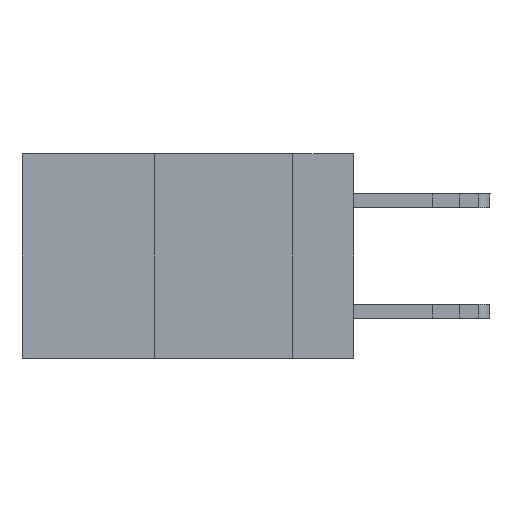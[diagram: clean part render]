
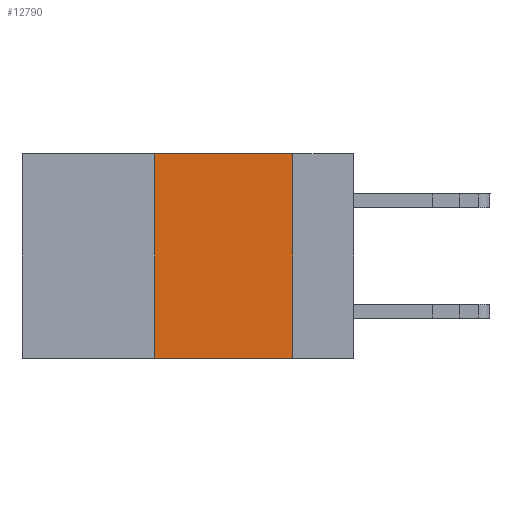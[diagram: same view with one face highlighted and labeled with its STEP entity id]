
A CAD part, left-side view. The second image highlights one B-rep face of the part: STEP entity #12790.
In plain terms, the highlighted planar face has unit normal (-1, 0, 0).
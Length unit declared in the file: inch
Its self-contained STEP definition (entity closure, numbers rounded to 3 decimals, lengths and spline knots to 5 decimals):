
#268 = CARTESIAN_POINT ( 'NONE',  ( 0., 0.36, 0. ) ) ;
#321 = FACE_OUTER_BOUND ( 'NONE', #9798, .T. ) ;
#323 = DIRECTION ( 'NONE',  ( 0., 0., 1. ) ) ;
#873 = ORIENTED_EDGE ( 'NONE', *, *, #4966, .F. ) ;
#1254 = EDGE_CURVE ( 'NONE', #4340, #8443, #14075, .T. ) ;
#1696 = EDGE_CURVE ( 'NONE', #13185, #4340, #14829, .T. ) ;
#3400 = LINE ( 'NONE', #268, #8341 ) ;
#4340 = VERTEX_POINT ( 'NONE', #11667 ) ;
#4399 = EDGE_CURVE ( 'NONE', #11257, #8443, #13982, .T. ) ;
#4766 = CARTESIAN_POINT ( 'NONE',  ( 0., 0.36, 0. ) ) ;
#4966 = EDGE_CURVE ( 'NONE', #11257, #13185, #3400, .T. ) ;
#5517 = DIRECTION ( 'NONE',  ( 0., 0., -1. ) ) ;
#5596 = DIRECTION ( 'NONE',  ( 1., 0., 0. ) ) ;
#7841 = VECTOR ( 'NONE', #8449, 39.37008 ) ;
#8010 = CARTESIAN_POINT ( 'NONE',  ( 0., 0.6, -0.37 ) ) ;
#8341 = VECTOR ( 'NONE', #323, 39.37008 ) ;
#8443 = VERTEX_POINT ( 'NONE', #10993 ) ;
#8449 = DIRECTION ( 'NONE',  ( 0., -1., 0. ) ) ;
#8572 = ORIENTED_EDGE ( 'NONE', *, *, #1696, .F. ) ;
#9428 = VECTOR ( 'NONE', #5517, 39.37008 ) ;
#9798 = EDGE_LOOP ( 'NONE', ( #14545, #8572, #873, #13237 ) ) ;
#10690 = VECTOR ( 'NONE', #12726, 39.37008 ) ;
#10721 = PLANE ( 'NONE',  #15469 ) ;
#10993 = CARTESIAN_POINT ( 'NONE',  ( 0., 0.11, -0.37 ) ) ;
#11257 = VERTEX_POINT ( 'NONE', #15049 ) ;
#11667 = CARTESIAN_POINT ( 'NONE',  ( 0., 0.11, 0. ) ) ;
#12030 = CARTESIAN_POINT ( 'NONE',  ( 0., 0.6, 0. ) ) ;
#12726 = DIRECTION ( 'NONE',  ( 0., -1., 0. ) ) ;
#12790 = ADVANCED_FACE ( 'NONE', ( #321 ), #10721, .F. ) ;
#13185 = VERTEX_POINT ( 'NONE', #4766 ) ;
#13237 = ORIENTED_EDGE ( 'NONE', *, *, #4399, .T. ) ;
#13553 = CARTESIAN_POINT ( 'NONE',  ( 0., 0.6, 0. ) ) ;
#13982 = LINE ( 'NONE', #8010, #10690 ) ;
#14075 = LINE ( 'NONE', #15241, #9428 ) ;
#14545 = ORIENTED_EDGE ( 'NONE', *, *, #1254, .F. ) ;
#14829 = LINE ( 'NONE', #13553, #7841 ) ;
#15049 = CARTESIAN_POINT ( 'NONE',  ( 0., 0.36, -0.37 ) ) ;
#15241 = CARTESIAN_POINT ( 'NONE',  ( 0., 0.11, 0. ) ) ;
#15469 = AXIS2_PLACEMENT_3D ( 'NONE', #12030, #5596, #15522 ) ;
#15522 = DIRECTION ( 'NONE',  ( 0., 0., -1. ) ) ;
